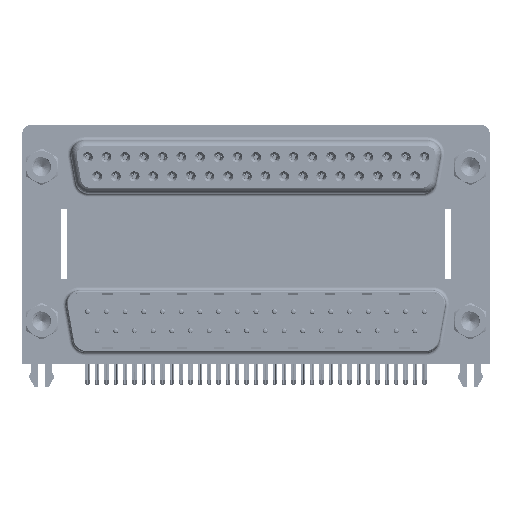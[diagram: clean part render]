
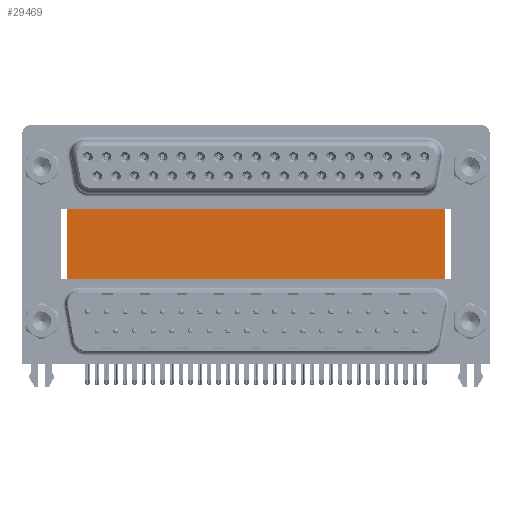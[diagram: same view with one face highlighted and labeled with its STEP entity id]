
A CAD part, top view. The second image highlights one B-rep face of the part: STEP entity #29469.
In plain terms, the highlighted planar face has unit normal (0, 0, 1).
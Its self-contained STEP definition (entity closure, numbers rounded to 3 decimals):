
#657 = CARTESIAN_POINT ( 'NONE',  ( 59.71, -3.735, -12. ) ) ;
#1164 = DIRECTION ( 'NONE',  ( 1., 0., 0. ) ) ;
#4736 = CARTESIAN_POINT ( 'NONE',  ( 3.79, 16.585, -12. ) ) ;
#6592 = ORIENTED_EDGE ( 'NONE', *, *, #35825, .T. ) ;
#10373 = LINE ( 'NONE', #56745, #48394 ) ;
#10432 = FACE_OUTER_BOUND ( 'NONE', #31145, .T. ) ;
#10600 = DIRECTION ( 'NONE',  ( 0., -1., 0. ) ) ;
#11188 = AXIS2_PLACEMENT_3D ( 'NONE', #4736, #27905, #51112 ) ;
#17279 = EDGE_CURVE ( 'NONE', #27226, #72827, #25748, .T. ) ;
#22386 = EDGE_CURVE ( 'NONE', #72827, #63246, #10373, .T. ) ;
#23992 = CARTESIAN_POINT ( 'NONE',  ( 3.79, -3.735, -12. ) ) ;
#25748 = LINE ( 'NONE', #48960, #63761 ) ;
#27226 = VERTEX_POINT ( 'NONE', #57806 ) ;
#27531 = LINE ( 'NONE', #23992, #45870 ) ;
#27905 = DIRECTION ( 'NONE',  ( 0., 0., -1. ) ) ;
#29469 = ADVANCED_FACE ( 'NONE', ( #10432 ), #40088, .F. ) ;
#30932 = ORIENTED_EDGE ( 'NONE', *, *, #22386, .F. ) ;
#31145 = EDGE_LOOP ( 'NONE', ( #66339, #30932, #37700, #6592 ) ) ;
#35825 = EDGE_CURVE ( 'NONE', #27226, #69984, #50516, .T. ) ;
#37700 = ORIENTED_EDGE ( 'NONE', *, *, #17279, .F. ) ;
#40088 = PLANE ( 'NONE',  #11188 ) ;
#45870 = VECTOR ( 'NONE', #1164, 1000. ) ;
#47461 = DIRECTION ( 'NONE',  ( 1., 0., 0. ) ) ;
#48394 = VECTOR ( 'NONE', #62814, 1000. ) ;
#48960 = CARTESIAN_POINT ( 'NONE',  ( 3.79, 16.585, -12. ) ) ;
#50516 = LINE ( 'NONE', #62653, #55688 ) ;
#51112 = DIRECTION ( 'NONE',  ( -1., 0., 0. ) ) ;
#55688 = VECTOR ( 'NONE', #10600, 1000. ) ;
#56745 = CARTESIAN_POINT ( 'NONE',  ( 59.71, 16.585, -12. ) ) ;
#57136 = EDGE_CURVE ( 'NONE', #69984, #63246, #27531, .T. ) ;
#57806 = CARTESIAN_POINT ( 'NONE',  ( 3.79, 16.585, -12. ) ) ;
#62653 = CARTESIAN_POINT ( 'NONE',  ( 3.79, 16.585, -12. ) ) ;
#62814 = DIRECTION ( 'NONE',  ( 0., -1., 0. ) ) ;
#63018 = CARTESIAN_POINT ( 'NONE',  ( 59.71, 16.585, -12. ) ) ;
#63246 = VERTEX_POINT ( 'NONE', #657 ) ;
#63761 = VECTOR ( 'NONE', #47461, 1000. ) ;
#66339 = ORIENTED_EDGE ( 'NONE', *, *, #57136, .T. ) ;
#69984 = VERTEX_POINT ( 'NONE', #71181 ) ;
#71181 = CARTESIAN_POINT ( 'NONE',  ( 3.79, -3.735, -12. ) ) ;
#72827 = VERTEX_POINT ( 'NONE', #63018 ) ;
